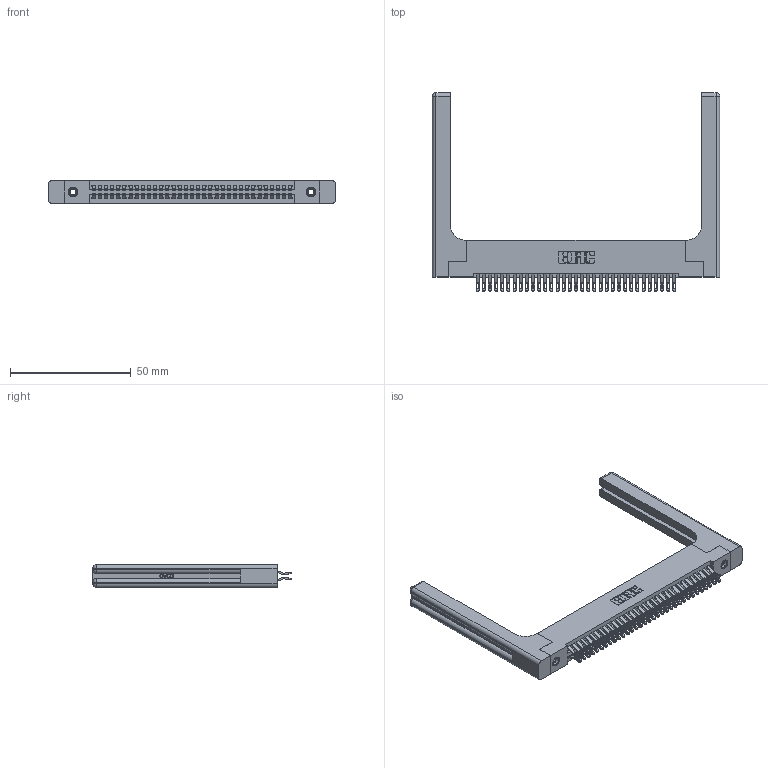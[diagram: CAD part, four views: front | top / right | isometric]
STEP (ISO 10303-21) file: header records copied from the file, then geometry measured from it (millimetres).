
FILE_DESCRIPTION (( 'STEP AP203' ), '1' );
FILE_NAME ('345-066-555-258.STEP', '2019-10-30T17:54:12', ( '' ), ( '' ), 'SwSTEP 2.0', 'SolidWorks 2016', '' );
FILE_SCHEMA (( 'CONFIG_CONTROL_DESIGN' ));
Length unit declared in the file: inch
Products named in the file (5): 345-250-001_345-250-001-102; 345-220-058_345-220-058; 345-292-001_555 Tail; 345-066-555-258; 345 Part_Flush Mounting Lugs - 0.156 Dia-TH
Assembly tree (71 placements, depth 2):
  345-066-555-258
    345 Part_Flush Mounting Lugs - 0.156 Dia-TH
    345-292-001_555 Tail  x66
    345-250-001_345-250-001-102  x2
    345-220-058_345-220-058  x2
Bounding box: 118.85 x 82.09 x 9.4 mm (x, y, z)
Volume: 20127.9 mm3; surface area: 22775.1 mm2
Topology: 71 solids, 71 shells, 4078 faces, 12689 edges, 8438 vertices
Faces by surface type: plane 2274, cylinder 1744, bspline 36, cone 12, sphere 8, torus 4
Entity records: 32612 total; most frequent: CARTESIAN_POINT 6503, ORIENTED_EDGE 5204, DIRECTION 4646, EDGE_CURVE 2602, LINE 2226, VECTOR 2226, VERTEX_POINT 1726, AXIS2_PLACEMENT_3D 1210
